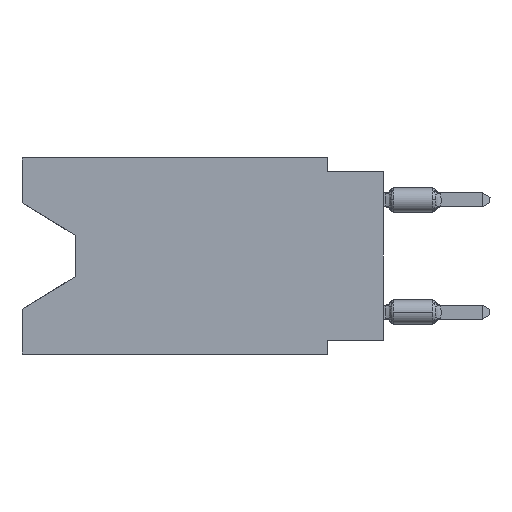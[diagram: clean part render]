
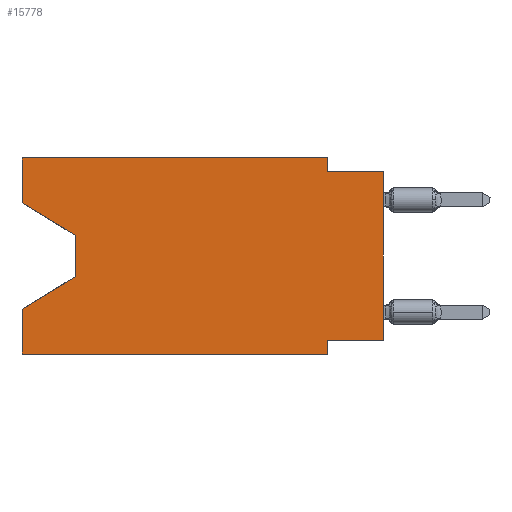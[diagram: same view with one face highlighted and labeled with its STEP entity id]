
A CAD part, left-side view. The second image highlights one B-rep face of the part: STEP entity #15778.
In plain terms, the highlighted planar face has unit normal (-1, 0, 0).
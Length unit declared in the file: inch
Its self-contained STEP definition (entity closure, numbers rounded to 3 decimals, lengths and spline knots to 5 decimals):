
#826 = CARTESIAN_POINT ( 'NONE',  ( 0., 0.1, -0.35 ) ) ;
#844 = CARTESIAN_POINT ( 'NONE',  ( 0., 0.645, 0. ) ) ;
#1023 = ORIENTED_EDGE ( 'NONE', *, *, #45015, .F. ) ;
#2334 = VECTOR ( 'NONE', #36158, 39.37008 ) ;
#2460 = VECTOR ( 'NONE', #5646, 39.37008 ) ;
#2529 = CARTESIAN_POINT ( 'NONE',  ( 0., 0.55, -0.138 ) ) ;
#2580 = EDGE_CURVE ( 'NONE', #40629, #15729, #20561, .T. ) ;
#3258 = CARTESIAN_POINT ( 'NONE',  ( 0., 0., -0.325 ) ) ;
#3514 = DIRECTION ( 'NONE',  ( 0., 0., -1. ) ) ;
#4157 = ORIENTED_EDGE ( 'NONE', *, *, #5568, .F. ) ;
#4185 = LINE ( 'NONE', #14782, #21954 ) ;
#4631 = VERTEX_POINT ( 'NONE', #44946 ) ;
#4656 = CARTESIAN_POINT ( 'NONE',  ( 0., 0.645, -0.26975 ) ) ;
#5044 = ORIENTED_EDGE ( 'NONE', *, *, #12805, .T. ) ;
#5276 = VECTOR ( 'NONE', #25817, 39.37008 ) ;
#5568 = EDGE_CURVE ( 'NONE', #32429, #45175, #14742, .T. ) ;
#5646 = DIRECTION ( 'NONE',  ( 0., -1., 0. ) ) ;
#6119 = CARTESIAN_POINT ( 'NONE',  ( 0., 0.645, 0. ) ) ;
#6476 = EDGE_LOOP ( 'NONE', ( #32665, #26889, #9574, #20542, #5044, #1023, #27835, #12373, #36500, #19866, #4157, #29216 ) ) ;
#6508 = EDGE_CURVE ( 'NONE', #40629, #34847, #16777, .T. ) ;
#6985 = VERTEX_POINT ( 'NONE', #25875 ) ;
#7482 = EDGE_CURVE ( 'NONE', #11367, #34847, #43545, .T. ) ;
#7761 = LINE ( 'NONE', #40041, #23907 ) ;
#9252 = AXIS2_PLACEMENT_3D ( 'NONE', #25650, #42235, #3514 ) ;
#9574 = ORIENTED_EDGE ( 'NONE', *, *, #22998, .T. ) ;
#10330 = CARTESIAN_POINT ( 'NONE',  ( 0., 0.1, 0. ) ) ;
#10434 = CARTESIAN_POINT ( 'NONE',  ( 0., 0.55, -0.212 ) ) ;
#10748 = VECTOR ( 'NONE', #26544, 39.37008 ) ;
#10954 = EDGE_CURVE ( 'NONE', #15133, #6985, #14709, .T. ) ;
#11034 = DIRECTION ( 'NONE',  ( 0., 0., 1. ) ) ;
#11367 = VERTEX_POINT ( 'NONE', #18917 ) ;
#12373 = ORIENTED_EDGE ( 'NONE', *, *, #6508, .T. ) ;
#12795 = CARTESIAN_POINT ( 'NONE',  ( 0., 0.645, -0.35 ) ) ;
#12805 = EDGE_CURVE ( 'NONE', #4631, #42132, #30749, .T. ) ;
#12846 = VECTOR ( 'NONE', #39601, 39.37008 ) ;
#13879 = DIRECTION ( 'NONE',  ( 0., 0.855, -0.519 ) ) ;
#14019 = CARTESIAN_POINT ( 'NONE',  ( 0., 0.645, 0. ) ) ;
#14070 = VECTOR ( 'NONE', #15136, 39.37008 ) ;
#14709 = LINE ( 'NONE', #36125, #12846 ) ;
#14742 = LINE ( 'NONE', #28352, #2334 ) ;
#14746 = VECTOR ( 'NONE', #13879, 39.37008 ) ;
#14782 = CARTESIAN_POINT ( 'NONE',  ( 0., 0.1, -0.35 ) ) ;
#15133 = VERTEX_POINT ( 'NONE', #2529 ) ;
#15136 = DIRECTION ( 'NONE',  ( 0., 0., 1. ) ) ;
#15729 = VERTEX_POINT ( 'NONE', #41323 ) ;
#15778 = ADVANCED_FACE ( 'NONE', ( #32542 ), #28413, .F. ) ;
#16003 = EDGE_CURVE ( 'NONE', #45175, #11367, #29998, .T. ) ;
#16355 = EDGE_CURVE ( 'NONE', #24911, #15133, #7761, .T. ) ;
#16777 = LINE ( 'NONE', #37741, #25984 ) ;
#17274 = LINE ( 'NONE', #844, #14070 ) ;
#18797 = VECTOR ( 'NONE', #11034, 39.37008 ) ;
#18917 = CARTESIAN_POINT ( 'NONE',  ( 0., 0.1, -0.025 ) ) ;
#19866 = ORIENTED_EDGE ( 'NONE', *, *, #16003, .F. ) ;
#20542 = ORIENTED_EDGE ( 'NONE', *, *, #29202, .F. ) ;
#20561 = LINE ( 'NONE', #3258, #45385 ) ;
#21852 = DIRECTION ( 'NONE',  ( 0., -0.855, -0.519 ) ) ;
#21954 = VECTOR ( 'NONE', #42456, 39.37008 ) ;
#21971 = VERTEX_POINT ( 'NONE', #4656 ) ;
#22998 = EDGE_CURVE ( 'NONE', #6985, #21971, #38320, .T. ) ;
#23802 = DIRECTION ( 'NONE',  ( 0., 1., 0. ) ) ;
#23907 = VECTOR ( 'NONE', #21852, 39.37008 ) ;
#24911 = VERTEX_POINT ( 'NONE', #31047 ) ;
#25250 = CARTESIAN_POINT ( 'NONE',  ( 0., 0., -0.325 ) ) ;
#25650 = CARTESIAN_POINT ( 'NONE',  ( 0., 0.645, 0. ) ) ;
#25817 = DIRECTION ( 'NONE',  ( 0., -1., 0. ) ) ;
#25875 = CARTESIAN_POINT ( 'NONE',  ( 0., 0.55, -0.212 ) ) ;
#25984 = VECTOR ( 'NONE', #30380, 39.37008 ) ;
#26215 = CARTESIAN_POINT ( 'NONE',  ( 0., 0., -0.025 ) ) ;
#26544 = DIRECTION ( 'NONE',  ( 0., 0., -1. ) ) ;
#26889 = ORIENTED_EDGE ( 'NONE', *, *, #10954, .T. ) ;
#27835 = ORIENTED_EDGE ( 'NONE', *, *, #2580, .F. ) ;
#28352 = CARTESIAN_POINT ( 'NONE',  ( 0., 0.645, 0. ) ) ;
#28413 = PLANE ( 'NONE',  #9252 ) ;
#29202 = EDGE_CURVE ( 'NONE', #4631, #21971, #36135, .T. ) ;
#29216 = ORIENTED_EDGE ( 'NONE', *, *, #34667, .F. ) ;
#29544 = CARTESIAN_POINT ( 'NONE',  ( 0., 0.1, 0. ) ) ;
#29998 = LINE ( 'NONE', #29544, #10748 ) ;
#30380 = DIRECTION ( 'NONE',  ( 0., 0., 1. ) ) ;
#30749 = LINE ( 'NONE', #12795, #2460 ) ;
#31047 = CARTESIAN_POINT ( 'NONE',  ( 0., 0.645, -0.08025 ) ) ;
#32429 = VERTEX_POINT ( 'NONE', #6119 ) ;
#32542 = FACE_OUTER_BOUND ( 'NONE', #6476, .T. ) ;
#32665 = ORIENTED_EDGE ( 'NONE', *, *, #16355, .T. ) ;
#34667 = EDGE_CURVE ( 'NONE', #24911, #32429, #17274, .T. ) ;
#34847 = VERTEX_POINT ( 'NONE', #26215 ) ;
#36125 = CARTESIAN_POINT ( 'NONE',  ( 0., 0.55, -0.138 ) ) ;
#36135 = LINE ( 'NONE', #14019, #18797 ) ;
#36158 = DIRECTION ( 'NONE',  ( 0., -1., 0. ) ) ;
#36500 = ORIENTED_EDGE ( 'NONE', *, *, #7482, .F. ) ;
#37741 = CARTESIAN_POINT ( 'NONE',  ( 0., 0., 0. ) ) ;
#38320 = LINE ( 'NONE', #10434, #14746 ) ;
#39601 = DIRECTION ( 'NONE',  ( 0., 0., -1. ) ) ;
#40041 = CARTESIAN_POINT ( 'NONE',  ( 0., 0.645, -0.08025 ) ) ;
#40099 = CARTESIAN_POINT ( 'NONE',  ( 0., 0., -0.025 ) ) ;
#40629 = VERTEX_POINT ( 'NONE', #25250 ) ;
#41323 = CARTESIAN_POINT ( 'NONE',  ( 0., 0.1, -0.325 ) ) ;
#42132 = VERTEX_POINT ( 'NONE', #826 ) ;
#42235 = DIRECTION ( 'NONE',  ( 1., 0., 0. ) ) ;
#42456 = DIRECTION ( 'NONE',  ( 0., 0., -1. ) ) ;
#43545 = LINE ( 'NONE', #40099, #5276 ) ;
#44946 = CARTESIAN_POINT ( 'NONE',  ( 0., 0.645, -0.35 ) ) ;
#45015 = EDGE_CURVE ( 'NONE', #15729, #42132, #4185, .T. ) ;
#45175 = VERTEX_POINT ( 'NONE', #10330 ) ;
#45385 = VECTOR ( 'NONE', #23802, 39.37008 ) ;
